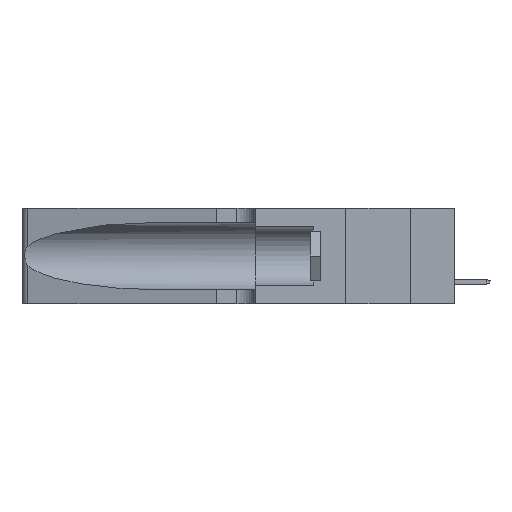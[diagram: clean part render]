
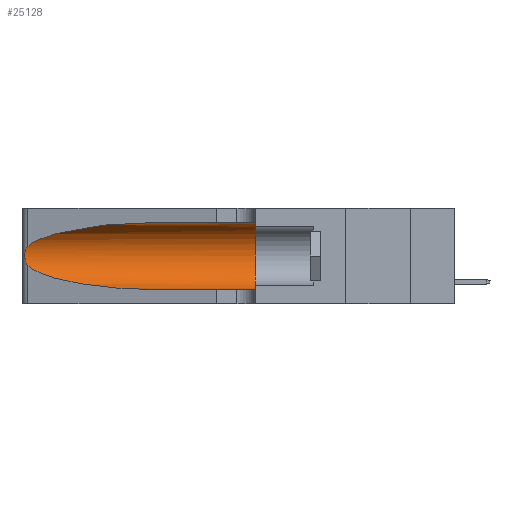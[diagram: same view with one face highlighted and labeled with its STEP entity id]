
A CAD part, left-side view. The second image highlights one B-rep face of the part: STEP entity #25128.
In plain terms, the highlighted cylindrical face has radius 3.308 mm (diameter 6.617 mm), a partial arc.
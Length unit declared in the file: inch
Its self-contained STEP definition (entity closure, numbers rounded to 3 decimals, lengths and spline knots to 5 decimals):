
#623 = ORIENTED_EDGE ( 'NONE', *, *, #14014, .T. ) ;
#1154 = CARTESIAN_POINT ( 'NONE',  ( 0.1305, 0.35, 0.185 ) ) ;
#1630 = CARTESIAN_POINT ( 'NONE',  ( 0.26075, 1.23896, 0.178 ) ) ;
#2127 = CARTESIAN_POINT ( 'NONE',  ( 0.1305, 0.72297, 0.05475 ) ) ;
#2680 = CARTESIAN_POINT ( 'NONE',  ( 0.18966, 0.96281, 0.05475 ) ) ;
#4919 = CARTESIAN_POINT ( 'NONE',  ( 0.18966, 0.96281, 0.31525 ) ) ;
#5384 = CARTESIAN_POINT ( 'NONE',  ( 0.1305, 1.61858, 0.185 ) ) ;
#6837 = EDGE_CURVE ( 'NONE', #27329, #22581, #18011, .T. ) ;
#7207 = ORIENTED_EDGE ( 'NONE', *, *, #13958, .T. ) ;
#7654 = VECTOR ( 'NONE', #21904, 39.37008 ) ;
#7698 = CARTESIAN_POINT ( 'NONE',  ( 0.26017, 1.23833, 0.17102 ) ) ;
#7870 = CARTESIAN_POINT ( 'NONE',  ( 0.1305, 0.35, 0.05475 ) ) ;
#9037 = EDGE_CURVE ( 'NONE', #11559, #20451, #15481, .T. ) ;
#9979 = ORIENTED_EDGE ( 'NONE', *, *, #16184, .F. ) ;
#10120 = CARTESIAN_POINT ( 'NONE',  ( 0.25856, 1.23593, 0.16098 ) ) ;
#10306 = CARTESIAN_POINT ( 'NONE',  ( 0.25789, 1.23486, 0.15765 ) ) ;
#10833 = ORIENTED_EDGE ( 'NONE', *, *, #6837, .F. ) ;
#11559 = VERTEX_POINT ( 'NONE', #28117 ) ;
#11974 = DIRECTION ( 'NONE',  ( 0., -1., 0. ) ) ;
#12429 = DIRECTION ( 'NONE',  ( 0., 0., 1. ) ) ;
#12903 = CARTESIAN_POINT ( 'NONE',  ( 0.25555, 1.22994, 0.2215 ) ) ;
#13081 = CARTESIAN_POINT ( 'NONE',  ( 0.25639, 1.23184, 0.21858 ) ) ;
#13258 = CARTESIAN_POINT ( 'NONE',  ( 0.25487, 1.22718, 0.22369 ) ) ;
#13699 = FACE_OUTER_BOUND ( 'NONE', #32976, .T. ) ;
#13958 = EDGE_CURVE ( 'NONE', #20451, #22581, #24145, .T. ) ;
#14014 = EDGE_CURVE ( 'NONE', #29689, #30095, #28195, .T. ) ;
#15481 =( BOUNDED_CURVE ( )  B_SPLINE_CURVE ( 3, ( #22259, #24645, #2680, #2127 ),
 .UNSPECIFIED., .F., .T. ) 
 B_SPLINE_CURVE_WITH_KNOTS ( ( 4, 4 ),
 ( 3.44316, 4.71239 ),
 .UNSPECIFIED. ) 
 CURVE ( )  GEOMETRIC_REPRESENTATION_ITEM ( )  RATIONAL_B_SPLINE_CURVE ( ( 1., 0.87, 0.87, 1. ) ) 
 REPRESENTATION_ITEM ( '' )  );
#15661 = CARTESIAN_POINT ( 'NONE',  ( 0.1305, 0.72297, 0.31525 ) ) ;
#15962 = LINE ( 'NONE', #19082, #18308 ) ;
#16184 = EDGE_CURVE ( 'NONE', #29689, #27329, #15962, .T. ) ;
#17422 = AXIS2_PLACEMENT_3D ( 'NONE', #1154, #23892, #12429 ) ;
#17509 = AXIS2_PLACEMENT_3D ( 'NONE', #5384, #11974, #31727 ) ;
#18011 = CIRCLE ( 'NONE', #17422, 0.13025 ) ;
#18308 = VECTOR ( 'NONE', #24619, 39.37008 ) ;
#18436 = CARTESIAN_POINT ( 'NONE',  ( 0.25854, 1.2359, 0.20912 ) ) ;
#19082 = CARTESIAN_POINT ( 'NONE',  ( 0.1305, 1.61858, 0.31525 ) ) ;
#19158 = CARTESIAN_POINT ( 'NONE',  ( 0.25555, 1.22993, 0.14849 ) ) ;
#20451 = VERTEX_POINT ( 'NONE', #22364 ) ;
#21397 = CARTESIAN_POINT ( 'NONE',  ( 0.25639, 1.23186, 0.15144 ) ) ;
#21558 = CARTESIAN_POINT ( 'NONE',  ( 0.25487, 1.22718, 0.22369 ) ) ;
#21904 = DIRECTION ( 'NONE',  ( 0., -1., 0. ) ) ;
#22259 = CARTESIAN_POINT ( 'NONE',  ( 0.25487, 1.22718, 0.14631 ) ) ;
#22364 = CARTESIAN_POINT ( 'NONE',  ( 0.1305, 0.72297, 0.05475 ) ) ;
#22581 = VERTEX_POINT ( 'NONE', #7870 ) ;
#23752 = CARTESIAN_POINT ( 'NONE',  ( 0.25487, 1.22718, 0.22369 ) ) ;
#23892 = DIRECTION ( 'NONE',  ( 0., 1., 0. ) ) ;
#24145 = LINE ( 'NONE', #32439, #7654 ) ;
#24619 = DIRECTION ( 'NONE',  ( 0., -1., 0. ) ) ;
#24645 = CARTESIAN_POINT ( 'NONE',  ( 0.2373, 1.15595, 0.08982 ) ) ;
#24716 = ORIENTED_EDGE ( 'NONE', *, *, #9037, .T. ) ;
#25128 = ADVANCED_FACE ( 'NONE', ( #13699 ), #31366, .F. ) ;
#25635 = CARTESIAN_POINT ( 'NONE',  ( 0.1305, 0.35, 0.31525 ) ) ;
#26921 = CARTESIAN_POINT ( 'NONE',  ( 0.1305, 0.72297, 0.31525 ) ) ;
#27329 = VERTEX_POINT ( 'NONE', #25635 ) ;
#28117 = CARTESIAN_POINT ( 'NONE',  ( 0.25487, 1.22718, 0.14631 ) ) ;
#28195 =( BOUNDED_CURVE ( )  B_SPLINE_CURVE ( 3, ( #15661, #4919, #32629, #21558 ),
 .UNSPECIFIED., .F., .F. ) 
 B_SPLINE_CURVE_WITH_KNOTS ( ( 4, 4 ),
 ( 1.5708, 2.84003 ),
 .UNSPECIFIED. ) 
 CURVE ( )  GEOMETRIC_REPRESENTATION_ITEM ( )  RATIONAL_B_SPLINE_CURVE ( ( 1., 0.87, 0.87, 1. ) ) 
 REPRESENTATION_ITEM ( '' )  );
#28837 = B_SPLINE_CURVE_WITH_KNOTS ( 'NONE', 3,
 ( #13258, #12903, #13081, #30057, #18436, #35573, #32994, #1630, #7698, #10120, #10306, #21397, #19158, #32655 ),
 .UNSPECIFIED., .F., .F.,
 ( 4, 2, 2, 2, 2, 2, 4 ),
 ( 0., 0.00027, 0.00053, 0.00107, 0.0016, 0.00187, 0.00214 ),
 .UNSPECIFIED. ) ;
#29689 = VERTEX_POINT ( 'NONE', #26921 ) ;
#29883 = EDGE_CURVE ( 'NONE', #30095, #11559, #28837, .T. ) ;
#30057 = CARTESIAN_POINT ( 'NONE',  ( 0.25787, 1.23484, 0.2124 ) ) ;
#30095 = VERTEX_POINT ( 'NONE', #23752 ) ;
#31366 = CYLINDRICAL_SURFACE ( 'NONE', #17509, 0.13025 ) ;
#31718 = ORIENTED_EDGE ( 'NONE', *, *, #29883, .T. ) ;
#31727 = DIRECTION ( 'NONE',  ( 0., 0., -1. ) ) ;
#32439 = CARTESIAN_POINT ( 'NONE',  ( 0.1305, 1.61858, 0.05475 ) ) ;
#32629 = CARTESIAN_POINT ( 'NONE',  ( 0.2373, 1.15595, 0.28018 ) ) ;
#32655 = CARTESIAN_POINT ( 'NONE',  ( 0.25487, 1.22718, 0.14631 ) ) ;
#32976 = EDGE_LOOP ( 'NONE', ( #623, #31718, #24716, #7207, #10833, #9979 ) ) ;
#32994 = CARTESIAN_POINT ( 'NONE',  ( 0.26075, 1.23896, 0.19203 ) ) ;
#35573 = CARTESIAN_POINT ( 'NONE',  ( 0.26018, 1.23835, 0.19895 ) ) ;
